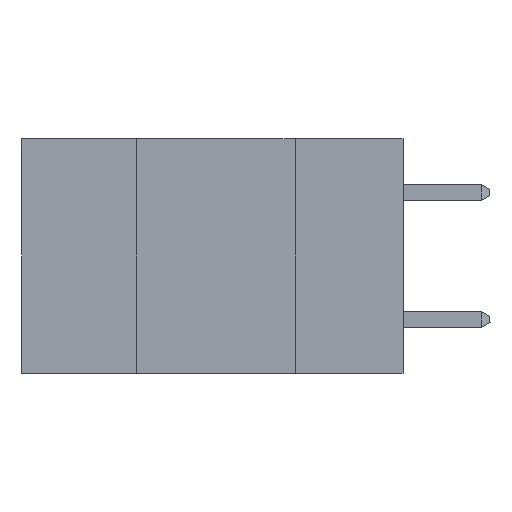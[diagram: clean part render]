
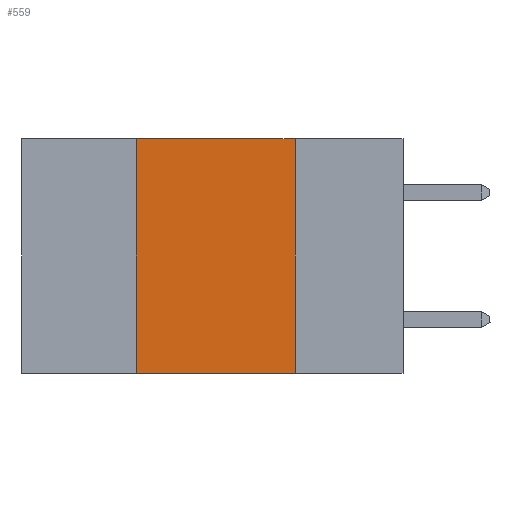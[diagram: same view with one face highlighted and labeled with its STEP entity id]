
A CAD part, left-side view. The second image highlights one B-rep face of the part: STEP entity #559.
In plain terms, the highlighted planar face has unit normal (-1, 0, 0).
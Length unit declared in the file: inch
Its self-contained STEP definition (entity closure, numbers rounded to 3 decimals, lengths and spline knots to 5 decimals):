
#559 = ADVANCED_FACE ( 'NONE', ( #19186 ), #14173, .F. ) ;
#1039 = CARTESIAN_POINT ( 'NONE',  ( 0., 0.6, -0.37 ) ) ;
#3677 = CARTESIAN_POINT ( 'NONE',  ( 0., 0.17, -0.37 ) ) ;
#3858 = CARTESIAN_POINT ( 'NONE',  ( 0., 0.42, -0.37 ) ) ;
#3956 = CARTESIAN_POINT ( 'NONE',  ( 0., 0.17, 0. ) ) ;
#4207 = ORIENTED_EDGE ( 'NONE', *, *, #19703, .F. ) ;
#4563 = ORIENTED_EDGE ( 'NONE', *, *, #23107, .F. ) ;
#4608 = ORIENTED_EDGE ( 'NONE', *, *, #12600, .F. ) ;
#4722 = ORIENTED_EDGE ( 'NONE', *, *, #7882, .T. ) ;
#5649 = VECTOR ( 'NONE', #9389, 39.37008 ) ;
#5824 = CARTESIAN_POINT ( 'NONE',  ( 0., 0.17, 0. ) ) ;
#7882 = EDGE_CURVE ( 'NONE', #22697, #9479, #17277, .T. ) ;
#8141 = CARTESIAN_POINT ( 'NONE',  ( 0., 0.42, 0. ) ) ;
#9389 = DIRECTION ( 'NONE',  ( 0., 0., -1. ) ) ;
#9479 = VERTEX_POINT ( 'NONE', #3677 ) ;
#9556 = DIRECTION ( 'NONE',  ( 1., 0., 0. ) ) ;
#9633 = VECTOR ( 'NONE', #22115, 39.37008 ) ;
#10040 = DIRECTION ( 'NONE',  ( 0., 0., -1. ) ) ;
#10339 = LINE ( 'NONE', #5824, #5649 ) ;
#11421 = VECTOR ( 'NONE', #20912, 39.37008 ) ;
#11583 = CARTESIAN_POINT ( 'NONE',  ( 0., 0.6, 0. ) ) ;
#11753 = CARTESIAN_POINT ( 'NONE',  ( 0., 0.6, 0. ) ) ;
#12600 = EDGE_CURVE ( 'NONE', #22697, #23126, #16162, .T. ) ;
#12668 = LINE ( 'NONE', #11583, #9633 ) ;
#12851 = VERTEX_POINT ( 'NONE', #3956 ) ;
#13669 = DIRECTION ( 'NONE',  ( 0., -1., 0. ) ) ;
#14173 = PLANE ( 'NONE',  #21618 ) ;
#16162 = LINE ( 'NONE', #19180, #11421 ) ;
#17277 = LINE ( 'NONE', #1039, #21865 ) ;
#19180 = CARTESIAN_POINT ( 'NONE',  ( 0., 0.42, 0. ) ) ;
#19186 = FACE_OUTER_BOUND ( 'NONE', #21569, .T. ) ;
#19703 = EDGE_CURVE ( 'NONE', #12851, #9479, #10339, .T. ) ;
#20912 = DIRECTION ( 'NONE',  ( 0., 0., 1. ) ) ;
#21569 = EDGE_LOOP ( 'NONE', ( #4207, #4563, #4608, #4722 ) ) ;
#21618 = AXIS2_PLACEMENT_3D ( 'NONE', #11753, #9556, #10040 ) ;
#21865 = VECTOR ( 'NONE', #13669, 39.37008 ) ;
#22115 = DIRECTION ( 'NONE',  ( 0., -1., 0. ) ) ;
#22697 = VERTEX_POINT ( 'NONE', #3858 ) ;
#23107 = EDGE_CURVE ( 'NONE', #23126, #12851, #12668, .T. ) ;
#23126 = VERTEX_POINT ( 'NONE', #8141 ) ;
